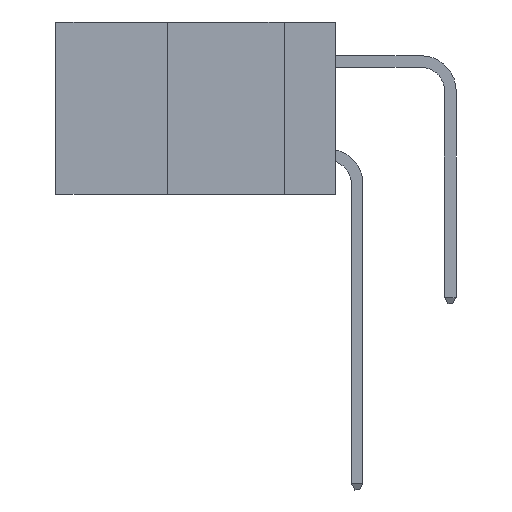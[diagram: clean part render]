
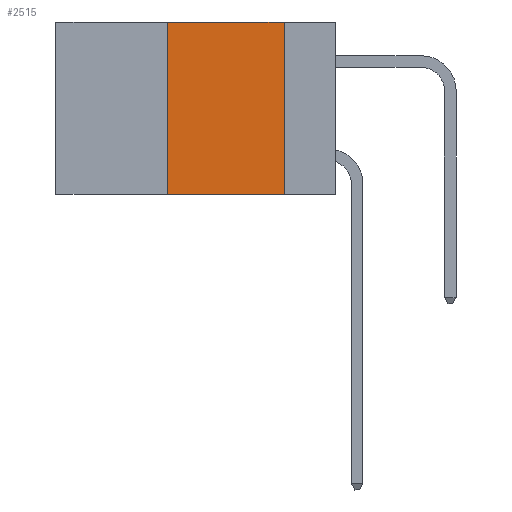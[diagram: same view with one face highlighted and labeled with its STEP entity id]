
A CAD part, left-side view. The second image highlights one B-rep face of the part: STEP entity #2515.
In plain terms, the highlighted planar face has unit normal (-1, 0, 0).
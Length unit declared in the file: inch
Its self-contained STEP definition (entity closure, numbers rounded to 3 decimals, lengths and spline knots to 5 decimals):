
#14 = DIRECTION ( 'NONE',  ( 0., 0., 1. ) ) ;
#450 = VECTOR ( 'NONE', #6246, 39.37008 ) ;
#1235 = LINE ( 'NONE', #10453, #450 ) ;
#1310 = VERTEX_POINT ( 'NONE', #3200 ) ;
#1929 = EDGE_LOOP ( 'NONE', ( #1932, #5751, #9550, #4878 ) ) ;
#1932 = ORIENTED_EDGE ( 'NONE', *, *, #2768, .F. ) ;
#2515 = ADVANCED_FACE ( 'NONE', ( #12905 ), #3782, .F. ) ;
#2768 = EDGE_CURVE ( 'NONE', #5778, #10554, #3166, .T. ) ;
#2892 = EDGE_CURVE ( 'NONE', #1310, #5778, #1235, .T. ) ;
#3166 = LINE ( 'NONE', #11443, #6038 ) ;
#3200 = CARTESIAN_POINT ( 'NONE',  ( 0., 0.36, 0. ) ) ;
#3218 = EDGE_CURVE ( 'NONE', #9444, #10554, #12055, .T. ) ;
#3782 = PLANE ( 'NONE',  #7210 ) ;
#4614 = VECTOR ( 'NONE', #14, 39.37008 ) ;
#4878 = ORIENTED_EDGE ( 'NONE', *, *, #3218, .T. ) ;
#5307 = CARTESIAN_POINT ( 'NONE',  ( 0., 0.11, -0.37 ) ) ;
#5751 = ORIENTED_EDGE ( 'NONE', *, *, #2892, .F. ) ;
#5778 = VERTEX_POINT ( 'NONE', #11152 ) ;
#6038 = VECTOR ( 'NONE', #10250, 39.37008 ) ;
#6246 = DIRECTION ( 'NONE',  ( 0., -1., 0. ) ) ;
#7210 = AXIS2_PLACEMENT_3D ( 'NONE', #11075, #13116, #7800 ) ;
#7800 = DIRECTION ( 'NONE',  ( 0., 0., -1. ) ) ;
#8389 = CARTESIAN_POINT ( 'NONE',  ( 0., 0.6, -0.37 ) ) ;
#8441 = DIRECTION ( 'NONE',  ( 0., -1., 0. ) ) ;
#8745 = LINE ( 'NONE', #13190, #4614 ) ;
#9444 = VERTEX_POINT ( 'NONE', #9584 ) ;
#9550 = ORIENTED_EDGE ( 'NONE', *, *, #9965, .F. ) ;
#9584 = CARTESIAN_POINT ( 'NONE',  ( 0., 0.36, -0.37 ) ) ;
#9965 = EDGE_CURVE ( 'NONE', #9444, #1310, #8745, .T. ) ;
#10250 = DIRECTION ( 'NONE',  ( 0., 0., -1. ) ) ;
#10453 = CARTESIAN_POINT ( 'NONE',  ( 0., 0.6, 0. ) ) ;
#10554 = VERTEX_POINT ( 'NONE', #5307 ) ;
#11075 = CARTESIAN_POINT ( 'NONE',  ( 0., 0.6, 0. ) ) ;
#11152 = CARTESIAN_POINT ( 'NONE',  ( 0., 0.11, 0. ) ) ;
#11443 = CARTESIAN_POINT ( 'NONE',  ( 0., 0.11, 0. ) ) ;
#12055 = LINE ( 'NONE', #8389, #13196 ) ;
#12905 = FACE_OUTER_BOUND ( 'NONE', #1929, .T. ) ;
#13116 = DIRECTION ( 'NONE',  ( 1., 0., 0. ) ) ;
#13190 = CARTESIAN_POINT ( 'NONE',  ( 0., 0.36, 0. ) ) ;
#13196 = VECTOR ( 'NONE', #8441, 39.37008 ) ;
